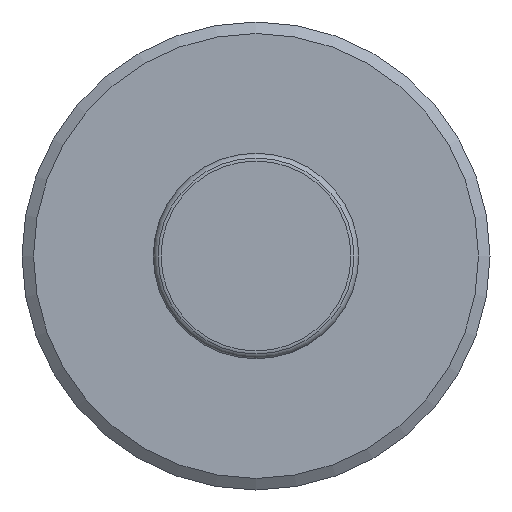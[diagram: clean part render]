
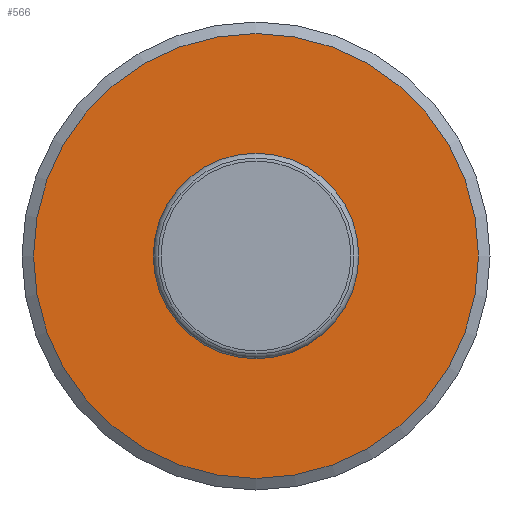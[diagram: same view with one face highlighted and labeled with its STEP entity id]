
A CAD part, front view. The second image highlights one B-rep face of the part: STEP entity #566.
In plain terms, the highlighted planar face has unit normal (0, -1, 0).
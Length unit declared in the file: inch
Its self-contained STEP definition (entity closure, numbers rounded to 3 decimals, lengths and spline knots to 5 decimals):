
#532=CARTESIAN_POINT('',(0.2272,0.,0.0));
#533=VERTEX_POINT('',#532);
#534=CARTESIAN_POINT('',(0.0,0.0,0.0));
#535=DIRECTION('',(0.0,-1.0,0.0));
#536=DIRECTION('',(1.0,0.0,0.0));
#537=AXIS2_PLACEMENT_3D('',#534,#535,#536);
#538=CIRCLE('',#537,0.2272);
#539=EDGE_CURVE('',#533,#533,#538,.T.);
#547=CARTESIAN_POINT('',(0.1661,0.,0.0));
#548=DIRECTION('',(0.0,-1.0,0.0));
#549=DIRECTION('',(0.0,0.0,-1.0));
#550=AXIS2_PLACEMENT_3D('',#547,#548,#549);
#551=PLANE('',#550);
#552=ORIENTED_EDGE('',*,*,#539,.T.);
#553=EDGE_LOOP('',(#552));
#554=FACE_OUTER_BOUND('',#553,.T.);
#555=CARTESIAN_POINT('',(0.105,0.0,0.0));
#556=VERTEX_POINT('',#555);
#557=CARTESIAN_POINT('',(0.0,0.0,0.0));
#558=DIRECTION('',(0.0,-1.0,0.0));
#559=DIRECTION('',(1.0,0.0,0.0));
#560=AXIS2_PLACEMENT_3D('',#557,#558,#559);
#561=CIRCLE('',#560,0.105);
#562=EDGE_CURVE('',#556,#556,#561,.T.);
#563=ORIENTED_EDGE('',*,*,#562,.F.);
#564=EDGE_LOOP('',(#563));
#565=FACE_BOUND('',#564,.T.);
#566=ADVANCED_FACE('',(#554,#565),#551,.T.);
